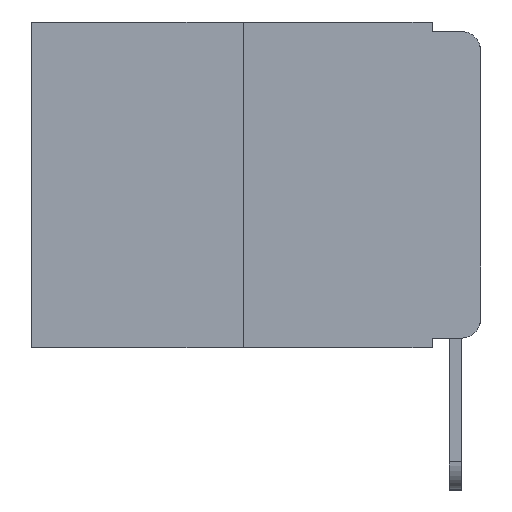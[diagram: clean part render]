
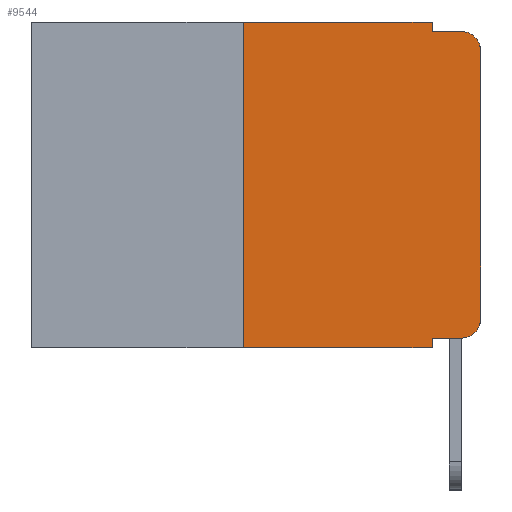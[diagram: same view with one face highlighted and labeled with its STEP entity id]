
A CAD part, left-side view. The second image highlights one B-rep face of the part: STEP entity #9544.
In plain terms, the highlighted planar face has unit normal (-1, 0, 0).
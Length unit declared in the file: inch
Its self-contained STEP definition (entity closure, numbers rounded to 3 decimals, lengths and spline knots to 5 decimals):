
#77 = ORIENTED_EDGE ( 'NONE', *, *, #2755, .T. ) ;
#172 = AXIS2_PLACEMENT_3D ( 'NONE', #11377, #5894, #12276 ) ;
#340 = VECTOR ( 'NONE', #7673, 39.37008 ) ;
#867 = VERTEX_POINT ( 'NONE', #5528 ) ;
#1147 = DIRECTION ( 'NONE',  ( 0., -1., 0. ) ) ;
#1582 = VERTEX_POINT ( 'NONE', #5184 ) ;
#2094 = VECTOR ( 'NONE', #3044, 39.37008 ) ;
#2234 = DIRECTION ( 'NONE',  ( 0., 0., -1. ) ) ;
#2276 = VECTOR ( 'NONE', #1147, 39.37008 ) ;
#2277 = CARTESIAN_POINT ( 'NONE',  ( 0., 0., -0.03 ) ) ;
#2346 = VERTEX_POINT ( 'NONE', #11340 ) ;
#2454 = LINE ( 'NONE', #9687, #2094 ) ;
#2750 = CARTESIAN_POINT ( 'NONE',  ( 0., 0.25, 0. ) ) ;
#2755 = EDGE_CURVE ( 'NONE', #2346, #6979, #8364, .T. ) ;
#2889 = CARTESIAN_POINT ( 'NONE',  ( 0., 0.473, 0. ) ) ;
#2899 = LINE ( 'NONE', #10180, #10150 ) ;
#3044 = DIRECTION ( 'NONE',  ( 0., -1., 0. ) ) ;
#3137 = DIRECTION ( 'NONE',  ( 0., 0., -1. ) ) ;
#3157 = CIRCLE ( 'NONE', #172, 0.02 ) ;
#3527 = DIRECTION ( 'NONE',  ( -1., 0., 0. ) ) ;
#3588 = EDGE_CURVE ( 'NONE', #1582, #7046, #2899, .T. ) ;
#3687 = ORIENTED_EDGE ( 'NONE', *, *, #9510, .F. ) ;
#3838 = EDGE_CURVE ( 'NONE', #8400, #9085, #7862, .T. ) ;
#3924 = DIRECTION ( 'NONE',  ( 0., -1., 0. ) ) ;
#3994 = ORIENTED_EDGE ( 'NONE', *, *, #8512, .F. ) ;
#4512 = VERTEX_POINT ( 'NONE', #5182 ) ;
#4896 = LINE ( 'NONE', #7163, #2276 ) ;
#5182 = CARTESIAN_POINT ( 'NONE',  ( 0., 0.02, -0.333 ) ) ;
#5184 = CARTESIAN_POINT ( 'NONE',  ( 0., 0.051, 0. ) ) ;
#5338 = VECTOR ( 'NONE', #6105, 39.37008 ) ;
#5454 = AXIS2_PLACEMENT_3D ( 'NONE', #10596, #8835, #3137 ) ;
#5528 = CARTESIAN_POINT ( 'NONE',  ( 0., 0.051, -0.333 ) ) ;
#5661 = DIRECTION ( 'NONE',  ( 0., 0., 1. ) ) ;
#5679 = EDGE_LOOP ( 'NONE', ( #8134, #8422, #3687, #11097, #3994, #6659, #77, #8271, #8545, #6968 ) ) ;
#5894 = DIRECTION ( 'NONE',  ( -1., 0., 0. ) ) ;
#6023 = PLANE ( 'NONE',  #5454 ) ;
#6105 = DIRECTION ( 'NONE',  ( 0., 0., 1. ) ) ;
#6157 = CARTESIAN_POINT ( 'NONE',  ( 0., 0.02, -0.01 ) ) ;
#6300 = CARTESIAN_POINT ( 'NONE',  ( 0., 0.051, -0.01 ) ) ;
#6659 = ORIENTED_EDGE ( 'NONE', *, *, #11072, .F. ) ;
#6957 = EDGE_CURVE ( 'NONE', #867, #6979, #7230, .T. ) ;
#6968 = ORIENTED_EDGE ( 'NONE', *, *, #10909, .T. ) ;
#6979 = VERTEX_POINT ( 'NONE', #10767 ) ;
#7046 = VERTEX_POINT ( 'NONE', #6300 ) ;
#7094 = CIRCLE ( 'NONE', #10137, 0.02 ) ;
#7098 = CARTESIAN_POINT ( 'NONE',  ( 0., 0.051, 0. ) ) ;
#7163 = CARTESIAN_POINT ( 'NONE',  ( 0., 0.051, -0.333 ) ) ;
#7170 = VERTEX_POINT ( 'NONE', #7347 ) ;
#7230 = LINE ( 'NONE', #7098, #9404 ) ;
#7347 = CARTESIAN_POINT ( 'NONE',  ( 0., 0.25, 0. ) ) ;
#7661 = EDGE_CURVE ( 'NONE', #9085, #7865, #3157, .T. ) ;
#7673 = DIRECTION ( 'NONE',  ( 0., -1., 0. ) ) ;
#7862 = LINE ( 'NONE', #9796, #5338 ) ;
#7865 = VERTEX_POINT ( 'NONE', #6157 ) ;
#8120 = LINE ( 'NONE', #2750, #9989 ) ;
#8134 = ORIENTED_EDGE ( 'NONE', *, *, #3838, .T. ) ;
#8271 = ORIENTED_EDGE ( 'NONE', *, *, #6957, .F. ) ;
#8364 = LINE ( 'NONE', #9327, #340 ) ;
#8400 = VERTEX_POINT ( 'NONE', #9428 ) ;
#8422 = ORIENTED_EDGE ( 'NONE', *, *, #7661, .T. ) ;
#8512 = EDGE_CURVE ( 'NONE', #7170, #1582, #11034, .T. ) ;
#8545 = ORIENTED_EDGE ( 'NONE', *, *, #9693, .T. ) ;
#8644 = VECTOR ( 'NONE', #3924, 39.37008 ) ;
#8835 = DIRECTION ( 'NONE',  ( 1., 0., 0. ) ) ;
#9085 = VERTEX_POINT ( 'NONE', #2277 ) ;
#9193 = CARTESIAN_POINT ( 'NONE',  ( 0., 0.02, -0.313 ) ) ;
#9327 = CARTESIAN_POINT ( 'NONE',  ( 0., 0.473, -0.343 ) ) ;
#9404 = VECTOR ( 'NONE', #2234, 39.37008 ) ;
#9428 = CARTESIAN_POINT ( 'NONE',  ( 0., 0., -0.313 ) ) ;
#9510 = EDGE_CURVE ( 'NONE', #7046, #7865, #2454, .T. ) ;
#9544 = ADVANCED_FACE ( 'NONE', ( #11846 ), #6023, .F. ) ;
#9687 = CARTESIAN_POINT ( 'NONE',  ( 0., 0.051, -0.01 ) ) ;
#9693 = EDGE_CURVE ( 'NONE', #867, #4512, #4896, .T. ) ;
#9796 = CARTESIAN_POINT ( 'NONE',  ( 0., 0., 0. ) ) ;
#9989 = VECTOR ( 'NONE', #5661, 39.37008 ) ;
#10095 = DIRECTION ( 'NONE',  ( 0., 0., -1. ) ) ;
#10137 = AXIS2_PLACEMENT_3D ( 'NONE', #9193, #3527, #10095 ) ;
#10150 = VECTOR ( 'NONE', #10531, 39.37008 ) ;
#10180 = CARTESIAN_POINT ( 'NONE',  ( 0., 0.051, 0. ) ) ;
#10531 = DIRECTION ( 'NONE',  ( 0., 0., -1. ) ) ;
#10596 = CARTESIAN_POINT ( 'NONE',  ( 0., 0.473, 0. ) ) ;
#10767 = CARTESIAN_POINT ( 'NONE',  ( 0., 0.051, -0.343 ) ) ;
#10909 = EDGE_CURVE ( 'NONE', #4512, #8400, #7094, .T. ) ;
#11034 = LINE ( 'NONE', #2889, #8644 ) ;
#11072 = EDGE_CURVE ( 'NONE', #2346, #7170, #8120, .T. ) ;
#11097 = ORIENTED_EDGE ( 'NONE', *, *, #3588, .F. ) ;
#11340 = CARTESIAN_POINT ( 'NONE',  ( 0., 0.25, -0.343 ) ) ;
#11377 = CARTESIAN_POINT ( 'NONE',  ( 0., 0.02, -0.03 ) ) ;
#11846 = FACE_OUTER_BOUND ( 'NONE', #5679, .T. ) ;
#12276 = DIRECTION ( 'NONE',  ( 0., 0., -1. ) ) ;
